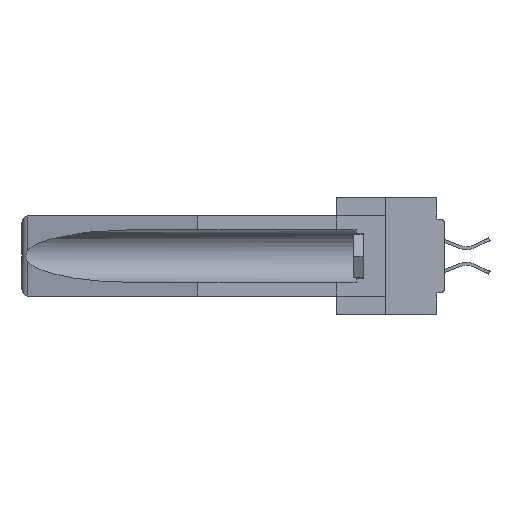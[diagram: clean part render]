
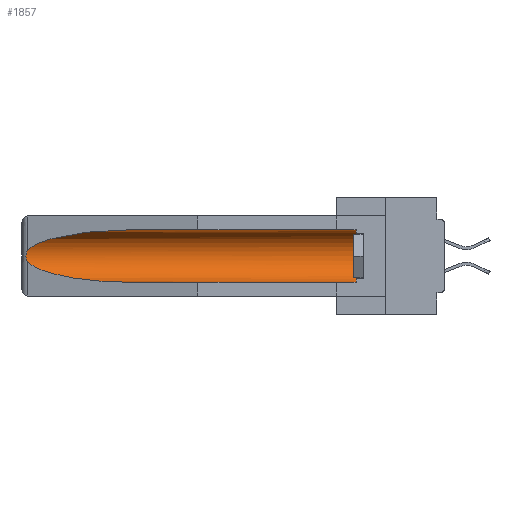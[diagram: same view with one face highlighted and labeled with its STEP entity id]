
A CAD part, left-side view. The second image highlights one B-rep face of the part: STEP entity #1857.
In plain terms, the highlighted cylindrical face has radius 2.857 mm (diameter 5.715 mm), a partial arc.
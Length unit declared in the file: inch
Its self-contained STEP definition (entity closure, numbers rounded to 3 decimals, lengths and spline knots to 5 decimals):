
#51 =( BOUNDED_CURVE ( )  B_SPLINE_CURVE ( 3, ( #28870, #1108, #32018, #32420 ),
 .UNSPECIFIED., .F., .F. ) 
 B_SPLINE_CURVE_WITH_KNOTS ( ( 4, 4 ),
 ( 4.71239, 6.08839 ),
 .UNSPECIFIED. ) 
 CURVE ( )  GEOMETRIC_REPRESENTATION_ITEM ( )  RATIONAL_B_SPLINE_CURVE ( ( 1., 0.848, 0.848, 1. ) ) 
 REPRESENTATION_ITEM ( '' )  );
#453 = CARTESIAN_POINT ( 'NONE',  ( 0.26655, 1.53094, -0.18657 ) ) ;
#580 = CARTESIAN_POINT ( 'NONE',  ( 0.2673, 1.53269, -0.17917 ) ) ;
#724 = VERTEX_POINT ( 'NONE', #33364 ) ;
#1108 = CARTESIAN_POINT ( 'NONE',  ( 0.21114, 1.30732, -0.059 ) ) ;
#1801 = ORIENTED_EDGE ( 'NONE', *, *, #19857, .T. ) ;
#1857 = ADVANCED_FACE ( 'NONE', ( #7660 ), #23290, .F. ) ;
#2454 = DIRECTION ( 'NONE',  ( 0., 0., 1. ) ) ;
#5682 = CARTESIAN_POINT ( 'NONE',  ( 0.26537, 1.52718, -0.19328 ) ) ;
#5730 = EDGE_CURVE ( 'NONE', #29441, #17210, #15838, .T. ) ;
#6629 = DIRECTION ( 'NONE',  ( 0., 1., 0. ) ) ;
#6631 = CARTESIAN_POINT ( 'NONE',  ( 0.26537, 1.52718, -0.14972 ) ) ;
#7660 = FACE_OUTER_BOUND ( 'NONE', #27252, .T. ) ;
#7944 = DIRECTION ( 'NONE',  ( 0., 0., 1. ) ) ;
#9334 = VECTOR ( 'NONE', #38202, 39.37008 ) ;
#12401 = AXIS2_PLACEMENT_3D ( 'NONE', #39316, #13908, #7944 ) ;
#12616 = CARTESIAN_POINT ( 'NONE',  ( 0.26654, 1.53092, -0.15636 ) ) ;
#13451 = CARTESIAN_POINT ( 'NONE',  ( 0.155, -0.30754, -0.059 ) ) ;
#13581 = EDGE_CURVE ( 'NONE', #34902, #724, #51, .T. ) ;
#13602 = CIRCLE ( 'NONE', #13893, 0.1125 ) ;
#13893 = AXIS2_PLACEMENT_3D ( 'NONE', #40154, #36756, #2454 ) ;
#13908 = DIRECTION ( 'NONE',  ( 0., 1., 0. ) ) ;
#14157 = LINE ( 'NONE', #13451, #9334 ) ;
#14833 = CARTESIAN_POINT ( 'NONE',  ( 0.25451, 1.48313, -0.24835 ) ) ;
#15838 =( BOUNDED_CURVE ( )  B_SPLINE_CURVE ( 3, ( #5682, #14833, #30518, #20878 ),
 .UNSPECIFIED., .F., .F. ) 
 B_SPLINE_CURVE_WITH_KNOTS ( ( 4, 4 ),
 ( 0.1948, 1.5708 ),
 .UNSPECIFIED. ) 
 CURVE ( )  GEOMETRIC_REPRESENTATION_ITEM ( )  RATIONAL_B_SPLINE_CURVE ( ( 1., 0.848, 0.848, 1. ) ) 
 REPRESENTATION_ITEM ( '' )  );
#16054 = CARTESIAN_POINT ( 'NONE',  ( 0.2673, 1.5327, -0.16383 ) ) ;
#16716 = LINE ( 'NONE', #25316, #17189 ) ;
#17189 = VECTOR ( 'NONE', #6629, 39.37008 ) ;
#17210 = VERTEX_POINT ( 'NONE', #32819 ) ;
#18257 = CARTESIAN_POINT ( 'NONE',  ( 0.155, 0.126, -0.284 ) ) ;
#19213 = CARTESIAN_POINT ( 'NONE',  ( 0.2675, 1.53308, -0.16763 ) ) ;
#19336 = CARTESIAN_POINT ( 'NONE',  ( 0.2675, 1.53308, -0.17534 ) ) ;
#19857 = EDGE_CURVE ( 'NONE', #724, #29441, #35555, .T. ) ;
#20323 = CARTESIAN_POINT ( 'NONE',  ( 0.155, 1.07973, -0.059 ) ) ;
#20878 = CARTESIAN_POINT ( 'NONE',  ( 0.155, 1.07973, -0.284 ) ) ;
#21399 = ORIENTED_EDGE ( 'NONE', *, *, #26568, .F. ) ;
#22355 = CARTESIAN_POINT ( 'NONE',  ( 0.26597, 1.5296, -0.19026 ) ) ;
#22487 = CARTESIAN_POINT ( 'NONE',  ( 0.26537, 1.52718, -0.19328 ) ) ;
#23104 = ORIENTED_EDGE ( 'NONE', *, *, #13581, .T. ) ;
#23290 = CYLINDRICAL_SURFACE ( 'NONE', #12401, 0.1125 ) ;
#25316 = CARTESIAN_POINT ( 'NONE',  ( 0.155, -0.30754, -0.284 ) ) ;
#25470 = VERTEX_POINT ( 'NONE', #18257 ) ;
#26568 = EDGE_CURVE ( 'NONE', #25470, #17210, #16716, .T. ) ;
#26933 = ORIENTED_EDGE ( 'NONE', *, *, #35531, .T. ) ;
#27252 = EDGE_LOOP ( 'NONE', ( #23104, #1801, #31769, #21399, #28265, #26933 ) ) ;
#28265 = ORIENTED_EDGE ( 'NONE', *, *, #36311, .T. ) ;
#28870 = CARTESIAN_POINT ( 'NONE',  ( 0.155, 1.07973, -0.059 ) ) ;
#29441 = VERTEX_POINT ( 'NONE', #36639 ) ;
#30518 = CARTESIAN_POINT ( 'NONE',  ( 0.21114, 1.30732, -0.284 ) ) ;
#31331 = CARTESIAN_POINT ( 'NONE',  ( 0.26597, 1.52961, -0.15275 ) ) ;
#31769 = ORIENTED_EDGE ( 'NONE', *, *, #5730, .T. ) ;
#32018 = CARTESIAN_POINT ( 'NONE',  ( 0.25451, 1.48313, -0.09465 ) ) ;
#32151 = CARTESIAN_POINT ( 'NONE',  ( 0.155, 0.126, -0.059 ) ) ;
#32420 = CARTESIAN_POINT ( 'NONE',  ( 0.26537, 1.52718, -0.14972 ) ) ;
#32819 = CARTESIAN_POINT ( 'NONE',  ( 0.155, 1.07973, -0.284 ) ) ;
#33364 = CARTESIAN_POINT ( 'NONE',  ( 0.26537, 1.52718, -0.14972 ) ) ;
#34902 = VERTEX_POINT ( 'NONE', #20323 ) ;
#35531 = EDGE_CURVE ( 'NONE', #36594, #34902, #14157, .T. ) ;
#35555 = B_SPLINE_CURVE_WITH_KNOTS ( 'NONE', 3,
 ( #6631, #31331, #12616, #16054, #19213, #19336, #580, #453, #22355, #22487 ),
 .UNSPECIFIED., .F., .F.,
 ( 4, 2, 2, 2, 4 ),
 ( 0., 0.00029, 0.00058, 0.00087, 0.00117 ),
 .UNSPECIFIED. ) ;
#36311 = EDGE_CURVE ( 'NONE', #25470, #36594, #13602, .T. ) ;
#36594 = VERTEX_POINT ( 'NONE', #32151 ) ;
#36639 = CARTESIAN_POINT ( 'NONE',  ( 0.26537, 1.52718, -0.19328 ) ) ;
#36756 = DIRECTION ( 'NONE',  ( 0., -1., 0. ) ) ;
#38202 = DIRECTION ( 'NONE',  ( 0., 1., 0. ) ) ;
#39316 = CARTESIAN_POINT ( 'NONE',  ( 0.155, -0.30754, -0.1715 ) ) ;
#40154 = CARTESIAN_POINT ( 'NONE',  ( 0.155, 0.126, -0.1715 ) ) ;
